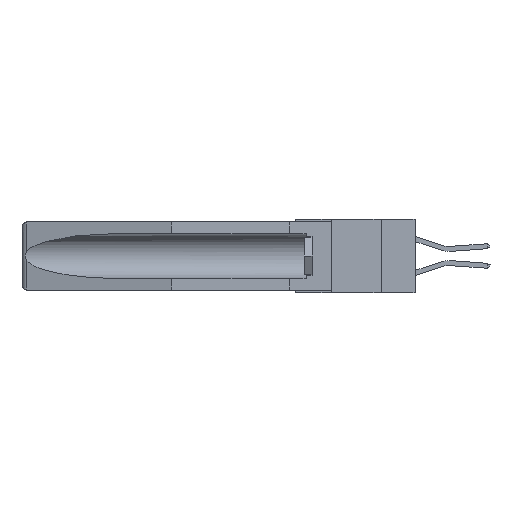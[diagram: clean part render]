
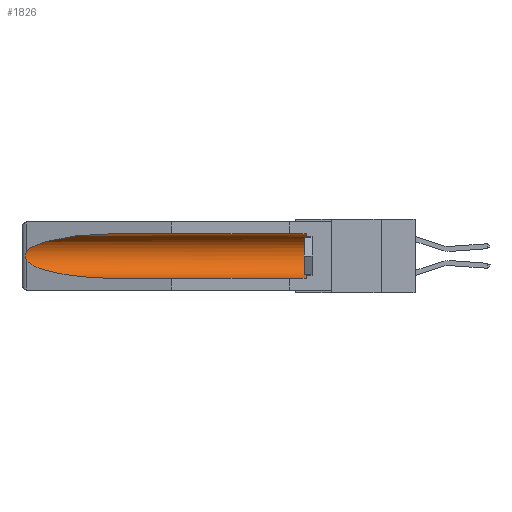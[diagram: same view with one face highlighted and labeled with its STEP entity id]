
A CAD part, left-side view. The second image highlights one B-rep face of the part: STEP entity #1826.
In plain terms, the highlighted cylindrical face has radius 2.857 mm (diameter 5.715 mm), a partial arc.
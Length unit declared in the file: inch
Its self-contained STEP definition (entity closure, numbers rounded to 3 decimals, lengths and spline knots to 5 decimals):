
#133 = ORIENTED_EDGE ( 'NONE', *, *, #19506, .T. ) ;
#501 = CARTESIAN_POINT ( 'NONE',  ( 0.26537, 1.52718, -0.14972 ) ) ;
#1063 = CARTESIAN_POINT ( 'NONE',  ( 0.2673, 1.5327, -0.16383 ) ) ;
#1316 = CARTESIAN_POINT ( 'NONE',  ( 0.26537, 1.52718, -0.14972 ) ) ;
#1826 = ADVANCED_FACE ( 'NONE', ( #9718 ), #3926, .F. ) ;
#3106 = VERTEX_POINT ( 'NONE', #23792 ) ;
#3169 = CARTESIAN_POINT ( 'NONE',  ( 0.26537, 1.52718, -0.19328 ) ) ;
#3266 = CARTESIAN_POINT ( 'NONE',  ( 0.2675, 1.53308, -0.16763 ) ) ;
#3926 = CYLINDRICAL_SURFACE ( 'NONE', #9223, 0.1125 ) ;
#4303 = CARTESIAN_POINT ( 'NONE',  ( 0.155, 0.126, -0.284 ) ) ;
#4571 = DIRECTION ( 'NONE',  ( 0., 1., 0. ) ) ;
#4906 = ORIENTED_EDGE ( 'NONE', *, *, #9617, .T. ) ;
#5347 = VERTEX_POINT ( 'NONE', #20790 ) ;
#5539 = DIRECTION ( 'NONE',  ( 0., 1., 0. ) ) ;
#6282 =( BOUNDED_CURVE ( )  B_SPLINE_CURVE ( 3, ( #26418, #15629, #9051, #501 ),
 .UNSPECIFIED., .F., .F. ) 
 B_SPLINE_CURVE_WITH_KNOTS ( ( 4, 4 ),
 ( 4.71239, 6.08839 ),
 .UNSPECIFIED. ) 
 CURVE ( )  GEOMETRIC_REPRESENTATION_ITEM ( )  RATIONAL_B_SPLINE_CURVE ( ( 1., 0.848, 0.848, 1. ) ) 
 REPRESENTATION_ITEM ( '' )  );
#6915 = AXIS2_PLACEMENT_3D ( 'NONE', #22445, #11659, #20062 ) ;
#8277 = DIRECTION ( 'NONE',  ( 0., 1., 0. ) ) ;
#9051 = CARTESIAN_POINT ( 'NONE',  ( 0.25451, 1.48313, -0.09465 ) ) ;
#9223 = AXIS2_PLACEMENT_3D ( 'NONE', #17231, #4571, #15137 ) ;
#9617 = EDGE_CURVE ( 'NONE', #10717, #13025, #27704, .T. ) ;
#9718 = FACE_OUTER_BOUND ( 'NONE', #22830, .T. ) ;
#10391 = CARTESIAN_POINT ( 'NONE',  ( 0.155, -0.30754, -0.059 ) ) ;
#10717 = VERTEX_POINT ( 'NONE', #17230 ) ;
#11659 = DIRECTION ( 'NONE',  ( 0., -1., 0. ) ) ;
#11857 = CIRCLE ( 'NONE', #6915, 0.1125 ) ;
#11943 = VECTOR ( 'NONE', #5539, 39.37008 ) ;
#11955 = CARTESIAN_POINT ( 'NONE',  ( 0.155, -0.30754, -0.284 ) ) ;
#12510 = CARTESIAN_POINT ( 'NONE',  ( 0.155, 1.07973, -0.284 ) ) ;
#13025 = VERTEX_POINT ( 'NONE', #22293 ) ;
#13258 = VERTEX_POINT ( 'NONE', #1316 ) ;
#14194 = VECTOR ( 'NONE', #8277, 39.37008 ) ;
#14630 = B_SPLINE_CURVE_WITH_KNOTS ( 'NONE', 3,
 ( #27077, #20348, #24750, #1063, #3266, #22541, #15909, #20538, #22730, #3169 ),
 .UNSPECIFIED., .F., .F.,
 ( 4, 2, 2, 2, 4 ),
 ( 0., 0.00029, 0.00058, 0.00087, 0.00117 ),
 .UNSPECIFIED. ) ;
#15137 = DIRECTION ( 'NONE',  ( 0., 0., 1. ) ) ;
#15222 = LINE ( 'NONE', #10391, #14194 ) ;
#15629 = CARTESIAN_POINT ( 'NONE',  ( 0.21114, 1.30732, -0.059 ) ) ;
#15909 = CARTESIAN_POINT ( 'NONE',  ( 0.2673, 1.53269, -0.17917 ) ) ;
#16483 = CARTESIAN_POINT ( 'NONE',  ( 0.21114, 1.30732, -0.284 ) ) ;
#16682 = EDGE_CURVE ( 'NONE', #5347, #13258, #6282, .T. ) ;
#17230 = CARTESIAN_POINT ( 'NONE',  ( 0.26537, 1.52718, -0.19328 ) ) ;
#17231 = CARTESIAN_POINT ( 'NONE',  ( 0.155, -0.30754, -0.1715 ) ) ;
#18076 = EDGE_CURVE ( 'NONE', #21205, #13025, #24838, .T. ) ;
#19506 = EDGE_CURVE ( 'NONE', #21205, #3106, #11857, .T. ) ;
#19616 = EDGE_CURVE ( 'NONE', #3106, #5347, #15222, .T. ) ;
#20062 = DIRECTION ( 'NONE',  ( 0., 0., 1. ) ) ;
#20348 = CARTESIAN_POINT ( 'NONE',  ( 0.26597, 1.52961, -0.15275 ) ) ;
#20374 = ORIENTED_EDGE ( 'NONE', *, *, #18076, .F. ) ;
#20538 = CARTESIAN_POINT ( 'NONE',  ( 0.26655, 1.53094, -0.18657 ) ) ;
#20790 = CARTESIAN_POINT ( 'NONE',  ( 0.155, 1.07973, -0.059 ) ) ;
#21205 = VERTEX_POINT ( 'NONE', #4303 ) ;
#21973 = ORIENTED_EDGE ( 'NONE', *, *, #26493, .T. ) ;
#22293 = CARTESIAN_POINT ( 'NONE',  ( 0.155, 1.07973, -0.284 ) ) ;
#22445 = CARTESIAN_POINT ( 'NONE',  ( 0.155, 0.126, -0.1715 ) ) ;
#22541 = CARTESIAN_POINT ( 'NONE',  ( 0.2675, 1.53308, -0.17534 ) ) ;
#22730 = CARTESIAN_POINT ( 'NONE',  ( 0.26597, 1.5296, -0.19026 ) ) ;
#22830 = EDGE_LOOP ( 'NONE', ( #27710, #21973, #4906, #20374, #133, #25500 ) ) ;
#23792 = CARTESIAN_POINT ( 'NONE',  ( 0.155, 0.126, -0.059 ) ) ;
#24750 = CARTESIAN_POINT ( 'NONE',  ( 0.26654, 1.53092, -0.15636 ) ) ;
#24838 = LINE ( 'NONE', #11955, #11943 ) ;
#25318 = CARTESIAN_POINT ( 'NONE',  ( 0.25451, 1.48313, -0.24835 ) ) ;
#25500 = ORIENTED_EDGE ( 'NONE', *, *, #19616, .T. ) ;
#26418 = CARTESIAN_POINT ( 'NONE',  ( 0.155, 1.07973, -0.059 ) ) ;
#26493 = EDGE_CURVE ( 'NONE', #13258, #10717, #14630, .T. ) ;
#27077 = CARTESIAN_POINT ( 'NONE',  ( 0.26537, 1.52718, -0.14972 ) ) ;
#27575 = CARTESIAN_POINT ( 'NONE',  ( 0.26537, 1.52718, -0.19328 ) ) ;
#27704 =( BOUNDED_CURVE ( )  B_SPLINE_CURVE ( 3, ( #27575, #25318, #16483, #12510 ),
 .UNSPECIFIED., .F., .F. ) 
 B_SPLINE_CURVE_WITH_KNOTS ( ( 4, 4 ),
 ( 0.1948, 1.5708 ),
 .UNSPECIFIED. ) 
 CURVE ( )  GEOMETRIC_REPRESENTATION_ITEM ( )  RATIONAL_B_SPLINE_CURVE ( ( 1., 0.848, 0.848, 1. ) ) 
 REPRESENTATION_ITEM ( '' )  );
#27710 = ORIENTED_EDGE ( 'NONE', *, *, #16682, .T. ) ;
